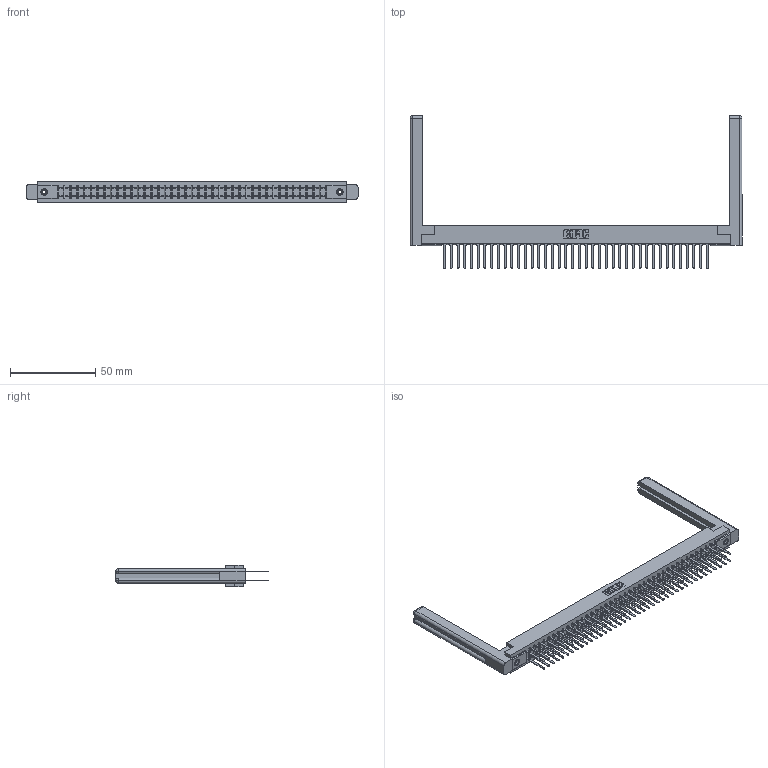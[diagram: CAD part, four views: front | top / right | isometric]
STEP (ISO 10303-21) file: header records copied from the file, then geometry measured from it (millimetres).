
FILE_DESCRIPTION (( 'STEP AP203' ), '1' );
FILE_NAME ('307-080-542-258.STEP', '2019-09-06T23:56:00', ( '' ), ( '' ), 'SwSTEP 2.0', 'SolidWorks 2016', '' );
FILE_SCHEMA (( 'CONFIG_CONTROL_DESIGN' ));
Length unit declared in the file: inch
Products named in the file (5): 345-250-001_345-250-001-102; 307-290-001_542; 307-080-542-258; 307 Part_.156 Dia Mounting Holes; 307-220-058
Assembly tree (85 placements, depth 2):
  307-080-542-258
    307 Part_.156 Dia Mounting Holes
    307-290-001_542  x80
    307-220-058  x2
    345-250-001_345-250-001-102  x2
Bounding box: 195.12 x 89.74 x 12.7 mm (x, y, z)
Volume: 28169.8 mm3; surface area: 32342.1 mm2
Topology: 85 solids, 85 shells, 3981 faces, 11077 edges, 7154 vertices
Faces by surface type: plane 2634, cylinder 1241, sphere 82, torus 12, cone 12
Entity records: 38419 total; most frequent: CARTESIAN_POINT 6303, ORIENTED_EDGE 6188, DIRECTION 6132, EDGE_CURVE 3094, VECTOR 2370, LINE 2370, VERTEX_POINT 1998, AXIS2_PLACEMENT_3D 1881
